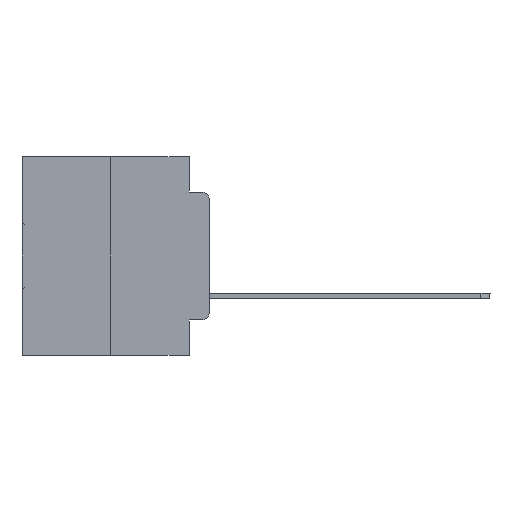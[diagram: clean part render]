
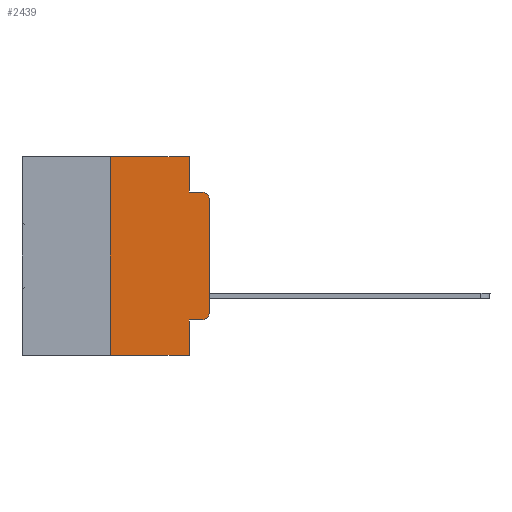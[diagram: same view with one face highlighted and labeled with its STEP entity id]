
A CAD part, left-side view. The second image highlights one B-rep face of the part: STEP entity #2439.
In plain terms, the highlighted planar face has unit normal (-1, 0, 0).
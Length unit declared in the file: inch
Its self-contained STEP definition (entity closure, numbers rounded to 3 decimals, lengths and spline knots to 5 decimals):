
#119 = LINE ( 'NONE', #10859, #24668 ) ;
#430 = CARTESIAN_POINT ( 'NONE',  ( 0., 0.25, 0. ) ) ;
#850 = DIRECTION ( 'NONE',  ( 0., -1., 0. ) ) ;
#919 = CARTESIAN_POINT ( 'NONE',  ( 0., 0.473, -0.5 ) ) ;
#1735 = LINE ( 'NONE', #7477, #21128 ) ;
#2292 = VERTEX_POINT ( 'NONE', #6054 ) ;
#2439 = ADVANCED_FACE ( 'NONE', ( #8672 ), #25733, .F. ) ;
#2966 = VERTEX_POINT ( 'NONE', #5952 ) ;
#3738 = CARTESIAN_POINT ( 'NONE',  ( 0., 0.25, -0.5 ) ) ;
#3951 = LINE ( 'NONE', #919, #22948 ) ;
#4386 = ORIENTED_EDGE ( 'NONE', *, *, #25436, .T. ) ;
#4997 = VECTOR ( 'NONE', #17224, 39.37008 ) ;
#5087 = DIRECTION ( 'NONE',  ( 0., -1., 0. ) ) ;
#5286 = ORIENTED_EDGE ( 'NONE', *, *, #5593, .F. ) ;
#5302 = CARTESIAN_POINT ( 'NONE',  ( 0., 0.051, -0.0885 ) ) ;
#5548 = CARTESIAN_POINT ( 'NONE',  ( 0., 0.051, -0.0885 ) ) ;
#5593 = EDGE_CURVE ( 'NONE', #24604, #2292, #11898, .T. ) ;
#5870 = AXIS2_PLACEMENT_3D ( 'NONE', #28620, #14384, #14190 ) ;
#5952 = CARTESIAN_POINT ( 'NONE',  ( 0., 0., -0.3915 ) ) ;
#6054 = CARTESIAN_POINT ( 'NONE',  ( 0., 0.051, -0.5 ) ) ;
#6306 = EDGE_CURVE ( 'NONE', #25974, #24850, #23585, .T. ) ;
#6776 = ORIENTED_EDGE ( 'NONE', *, *, #7653, .F. ) ;
#6847 = CARTESIAN_POINT ( 'NONE',  ( 0., 0.02, -0.0885 ) ) ;
#7036 = DIRECTION ( 'NONE',  ( 0., 0., -1. ) ) ;
#7366 = DIRECTION ( 'NONE',  ( 0., -1., 0. ) ) ;
#7477 = CARTESIAN_POINT ( 'NONE',  ( 0., 0.473, 0. ) ) ;
#7653 = EDGE_CURVE ( 'NONE', #8210, #29380, #14276, .T. ) ;
#7729 = ORIENTED_EDGE ( 'NONE', *, *, #16392, .F. ) ;
#7953 = CARTESIAN_POINT ( 'NONE',  ( 0., 0.02, -0.1085 ) ) ;
#8148 = VERTEX_POINT ( 'NONE', #21662 ) ;
#8151 = CARTESIAN_POINT ( 'NONE',  ( 0., 0.051, -0.4115 ) ) ;
#8210 = VERTEX_POINT ( 'NONE', #5302 ) ;
#8672 = FACE_OUTER_BOUND ( 'NONE', #14508, .T. ) ;
#9214 = DIRECTION ( 'NONE',  ( -1., 0., 0. ) ) ;
#9558 = CIRCLE ( 'NONE', #11283, 0.02 ) ;
#9572 = VERTEX_POINT ( 'NONE', #11203 ) ;
#9929 = CARTESIAN_POINT ( 'NONE',  ( 0., 0., 0. ) ) ;
#10859 = CARTESIAN_POINT ( 'NONE',  ( 0., 0.051, 0. ) ) ;
#11203 = CARTESIAN_POINT ( 'NONE',  ( 0., 0.051, 0. ) ) ;
#11276 = EDGE_CURVE ( 'NONE', #25974, #2292, #3951, .T. ) ;
#11283 = AXIS2_PLACEMENT_3D ( 'NONE', #25641, #9214, #28035 ) ;
#11898 = LINE ( 'NONE', #25657, #26026 ) ;
#12742 = DIRECTION ( 'NONE',  ( 0., 0., -1. ) ) ;
#12821 = EDGE_CURVE ( 'NONE', #29640, #29380, #13495, .T. ) ;
#12925 = ORIENTED_EDGE ( 'NONE', *, *, #11276, .T. ) ;
#13495 = CIRCLE ( 'NONE', #28955, 0.02 ) ;
#14190 = DIRECTION ( 'NONE',  ( 0., 0., -1. ) ) ;
#14276 = LINE ( 'NONE', #5548, #26905 ) ;
#14384 = DIRECTION ( 'NONE',  ( 1., 0., 0. ) ) ;
#14508 = EDGE_LOOP ( 'NONE', ( #18755, #17308, #6776, #30097, #7729, #20634, #12925, #5286, #4386, #18301 ) ) ;
#14936 = CARTESIAN_POINT ( 'NONE',  ( 0., 0., -0.1085 ) ) ;
#15246 = DIRECTION ( 'NONE',  ( 0., 0., -1. ) ) ;
#15254 = LINE ( 'NONE', #18456, #20867 ) ;
#16392 = EDGE_CURVE ( 'NONE', #24850, #9572, #1735, .T. ) ;
#17224 = DIRECTION ( 'NONE',  ( 0., 0., 1. ) ) ;
#17308 = ORIENTED_EDGE ( 'NONE', *, *, #12821, .T. ) ;
#18301 = ORIENTED_EDGE ( 'NONE', *, *, #27261, .T. ) ;
#18456 = CARTESIAN_POINT ( 'NONE',  ( 0., 0.051, -0.4115 ) ) ;
#18755 = ORIENTED_EDGE ( 'NONE', *, *, #21358, .T. ) ;
#19666 = EDGE_CURVE ( 'NONE', #9572, #8210, #119, .T. ) ;
#20634 = ORIENTED_EDGE ( 'NONE', *, *, #6306, .F. ) ;
#20867 = VECTOR ( 'NONE', #25321, 39.37008 ) ;
#21128 = VECTOR ( 'NONE', #5087, 39.37008 ) ;
#21358 = EDGE_CURVE ( 'NONE', #2966, #29640, #24188, .T. ) ;
#21662 = CARTESIAN_POINT ( 'NONE',  ( 0., 0.02, -0.4115 ) ) ;
#22317 = DIRECTION ( 'NONE',  ( -1., 0., 0. ) ) ;
#22343 = CARTESIAN_POINT ( 'NONE',  ( 0., 0.25, 0. ) ) ;
#22948 = VECTOR ( 'NONE', #7366, 39.37008 ) ;
#23585 = LINE ( 'NONE', #22343, #4997 ) ;
#24188 = LINE ( 'NONE', #9929, #28328 ) ;
#24604 = VERTEX_POINT ( 'NONE', #8151 ) ;
#24668 = VECTOR ( 'NONE', #12742, 39.37008 ) ;
#24850 = VERTEX_POINT ( 'NONE', #430 ) ;
#25321 = DIRECTION ( 'NONE',  ( 0., -1., 0. ) ) ;
#25436 = EDGE_CURVE ( 'NONE', #24604, #8148, #15254, .T. ) ;
#25641 = CARTESIAN_POINT ( 'NONE',  ( 0., 0.02, -0.3915 ) ) ;
#25657 = CARTESIAN_POINT ( 'NONE',  ( 0., 0.051, 0. ) ) ;
#25733 = PLANE ( 'NONE',  #5870 ) ;
#25974 = VERTEX_POINT ( 'NONE', #3738 ) ;
#26026 = VECTOR ( 'NONE', #7036, 39.37008 ) ;
#26905 = VECTOR ( 'NONE', #850, 39.37008 ) ;
#27261 = EDGE_CURVE ( 'NONE', #8148, #2966, #9558, .T. ) ;
#28035 = DIRECTION ( 'NONE',  ( 0., 0., -1. ) ) ;
#28328 = VECTOR ( 'NONE', #29158, 39.37008 ) ;
#28620 = CARTESIAN_POINT ( 'NONE',  ( 0., 0.473, 0. ) ) ;
#28955 = AXIS2_PLACEMENT_3D ( 'NONE', #7953, #22317, #15246 ) ;
#29158 = DIRECTION ( 'NONE',  ( 0., 0., 1. ) ) ;
#29380 = VERTEX_POINT ( 'NONE', #6847 ) ;
#29640 = VERTEX_POINT ( 'NONE', #14936 ) ;
#30097 = ORIENTED_EDGE ( 'NONE', *, *, #19666, .F. ) ;
